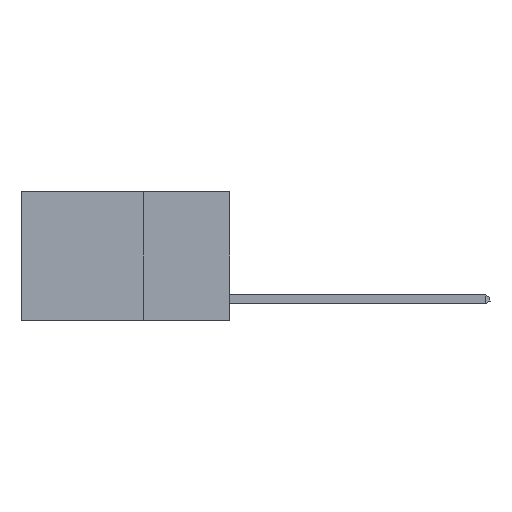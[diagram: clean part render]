
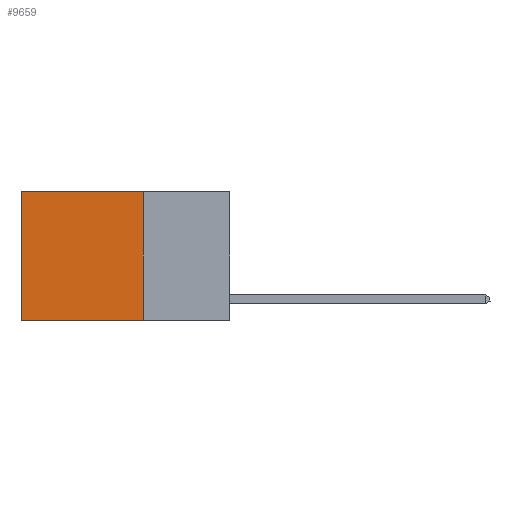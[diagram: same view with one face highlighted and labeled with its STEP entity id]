
A CAD part, left-side view. The second image highlights one B-rep face of the part: STEP entity #9659.
In plain terms, the highlighted planar face has unit normal (-1, 0, 0).
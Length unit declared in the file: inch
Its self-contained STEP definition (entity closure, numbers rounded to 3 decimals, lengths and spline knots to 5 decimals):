
#16 = CARTESIAN_POINT ( 'NONE',  ( 0.2625, 0.25, 0. ) ) ;
#364 = ORIENTED_EDGE ( 'NONE', *, *, #4335, .F. ) ;
#851 = ORIENTED_EDGE ( 'NONE', *, *, #3007, .F. ) ;
#1163 = VERTEX_POINT ( 'NONE', #2043 ) ;
#1198 = VERTEX_POINT ( 'NONE', #16 ) ;
#1548 = EDGE_CURVE ( 'NONE', #1163, #13328, #13421, .T. ) ;
#2037 = PLANE ( 'NONE',  #11983 ) ;
#2043 = CARTESIAN_POINT ( 'NONE',  ( 0.2625, 0.6, 0. ) ) ;
#2337 = DIRECTION ( 'NONE',  ( 0., 0., -1. ) ) ;
#3007 = EDGE_CURVE ( 'NONE', #7543, #13328, #6716, .T. ) ;
#3557 = VECTOR ( 'NONE', #10900, 39.37008 ) ;
#3975 = LINE ( 'NONE', #11039, #3557 ) ;
#4159 = EDGE_CURVE ( 'NONE', #1198, #1163, #10683, .T. ) ;
#4308 = FACE_OUTER_BOUND ( 'NONE', #13305, .T. ) ;
#4335 = EDGE_CURVE ( 'NONE', #1198, #7543, #3975, .T. ) ;
#4663 = VECTOR ( 'NONE', #11197, 39.37008 ) ;
#5943 = CARTESIAN_POINT ( 'NONE',  ( 0.2625, 0.6, -0.37 ) ) ;
#5991 = ORIENTED_EDGE ( 'NONE', *, *, #4159, .T. ) ;
#6615 = CARTESIAN_POINT ( 'NONE',  ( 0.2625, 0.6, 0. ) ) ;
#6627 = ORIENTED_EDGE ( 'NONE', *, *, #1548, .T. ) ;
#6716 = LINE ( 'NONE', #13880, #11996 ) ;
#7543 = VERTEX_POINT ( 'NONE', #10064 ) ;
#9659 = ADVANCED_FACE ( 'NONE', ( #4308 ), #2037, .F. ) ;
#10064 = CARTESIAN_POINT ( 'NONE',  ( 0.2625, 0.25, -0.37 ) ) ;
#10324 = DIRECTION ( 'NONE',  ( 1., 0., 0. ) ) ;
#10683 = LINE ( 'NONE', #12794, #13456 ) ;
#10900 = DIRECTION ( 'NONE',  ( 0., 0., -1. ) ) ;
#11039 = CARTESIAN_POINT ( 'NONE',  ( 0.2625, 0.25, 0. ) ) ;
#11197 = DIRECTION ( 'NONE',  ( 0., 0., -1. ) ) ;
#11983 = AXIS2_PLACEMENT_3D ( 'NONE', #13526, #10324, #2337 ) ;
#11996 = VECTOR ( 'NONE', #12723, 39.37008 ) ;
#12723 = DIRECTION ( 'NONE',  ( 0., 1., 0. ) ) ;
#12794 = CARTESIAN_POINT ( 'NONE',  ( 0.2625, 0.25, 0. ) ) ;
#13305 = EDGE_LOOP ( 'NONE', ( #6627, #851, #364, #5991 ) ) ;
#13328 = VERTEX_POINT ( 'NONE', #5943 ) ;
#13421 = LINE ( 'NONE', #6615, #4663 ) ;
#13456 = VECTOR ( 'NONE', #14027, 39.37008 ) ;
#13526 = CARTESIAN_POINT ( 'NONE',  ( 0.2625, 0.25, 0. ) ) ;
#13880 = CARTESIAN_POINT ( 'NONE',  ( 0.2625, 0.25, -0.37 ) ) ;
#14027 = DIRECTION ( 'NONE',  ( 0., 1., 0. ) ) ;
